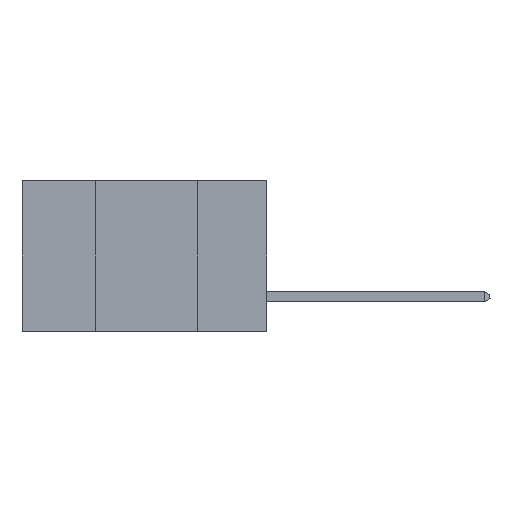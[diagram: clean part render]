
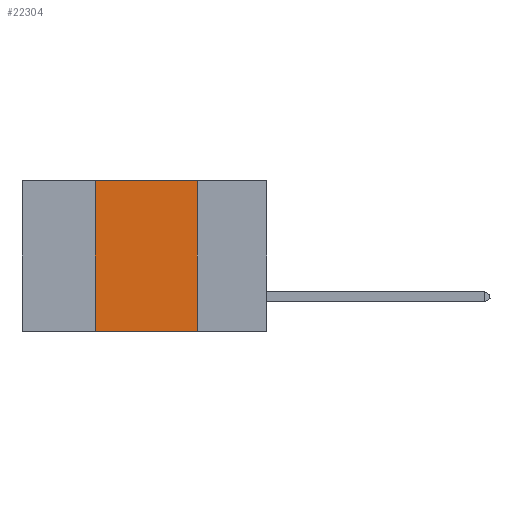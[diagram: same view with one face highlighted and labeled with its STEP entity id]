
A CAD part, left-side view. The second image highlights one B-rep face of the part: STEP entity #22304.
In plain terms, the highlighted planar face has unit normal (-1, 0, 0).
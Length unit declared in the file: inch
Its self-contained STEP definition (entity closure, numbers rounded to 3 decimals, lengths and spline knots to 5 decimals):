
#1137 = CARTESIAN_POINT ( 'NONE',  ( 0., 0.6, 0. ) ) ;
#4261 = VECTOR ( 'NONE', #34832, 39.37008 ) ;
#5614 = VERTEX_POINT ( 'NONE', #22439 ) ;
#7824 = DIRECTION ( 'NONE',  ( 1., 0., 0. ) ) ;
#8392 = EDGE_CURVE ( 'NONE', #9768, #23842, #9363, .T. ) ;
#9180 = EDGE_CURVE ( 'NONE', #9768, #5614, #40597, .T. ) ;
#9363 = LINE ( 'NONE', #10835, #46398 ) ;
#9768 = VERTEX_POINT ( 'NONE', #19124 ) ;
#10835 = CARTESIAN_POINT ( 'NONE',  ( 0., 0.42, 0. ) ) ;
#10965 = EDGE_LOOP ( 'NONE', ( #18289, #37311, #19542, #40049 ) ) ;
#12415 = CARTESIAN_POINT ( 'NONE',  ( 0., 0.17, 0. ) ) ;
#12876 = LINE ( 'NONE', #39255, #17415 ) ;
#16667 = CARTESIAN_POINT ( 'NONE',  ( 0., 0.6, -0.37 ) ) ;
#17415 = VECTOR ( 'NONE', #46601, 39.37008 ) ;
#18289 = ORIENTED_EDGE ( 'NONE', *, *, #31097, .F. ) ;
#19015 = VECTOR ( 'NONE', #39073, 39.37008 ) ;
#19124 = CARTESIAN_POINT ( 'NONE',  ( 0., 0.42, -0.37 ) ) ;
#19542 = ORIENTED_EDGE ( 'NONE', *, *, #8392, .F. ) ;
#21413 = LINE ( 'NONE', #34515, #4261 ) ;
#21854 = DIRECTION ( 'NONE',  ( 0., 0., 1. ) ) ;
#22304 = ADVANCED_FACE ( 'NONE', ( #46222 ), #40759, .F. ) ;
#22439 = CARTESIAN_POINT ( 'NONE',  ( 0., 0.17, -0.37 ) ) ;
#23842 = VERTEX_POINT ( 'NONE', #27764 ) ;
#26478 = DIRECTION ( 'NONE',  ( 0., 0., -1. ) ) ;
#27764 = CARTESIAN_POINT ( 'NONE',  ( 0., 0.42, 0. ) ) ;
#30371 = AXIS2_PLACEMENT_3D ( 'NONE', #1137, #7824, #26478 ) ;
#31097 = EDGE_CURVE ( 'NONE', #47053, #5614, #12876, .T. ) ;
#34515 = CARTESIAN_POINT ( 'NONE',  ( 0., 0.6, 0. ) ) ;
#34832 = DIRECTION ( 'NONE',  ( 0., -1., 0. ) ) ;
#34985 = EDGE_CURVE ( 'NONE', #23842, #47053, #21413, .T. ) ;
#37311 = ORIENTED_EDGE ( 'NONE', *, *, #34985, .F. ) ;
#39073 = DIRECTION ( 'NONE',  ( 0., -1., 0. ) ) ;
#39255 = CARTESIAN_POINT ( 'NONE',  ( 0., 0.17, 0. ) ) ;
#40049 = ORIENTED_EDGE ( 'NONE', *, *, #9180, .T. ) ;
#40597 = LINE ( 'NONE', #16667, #19015 ) ;
#40759 = PLANE ( 'NONE',  #30371 ) ;
#46222 = FACE_OUTER_BOUND ( 'NONE', #10965, .T. ) ;
#46398 = VECTOR ( 'NONE', #21854, 39.37008 ) ;
#46601 = DIRECTION ( 'NONE',  ( 0., 0., -1. ) ) ;
#47053 = VERTEX_POINT ( 'NONE', #12415 ) ;
